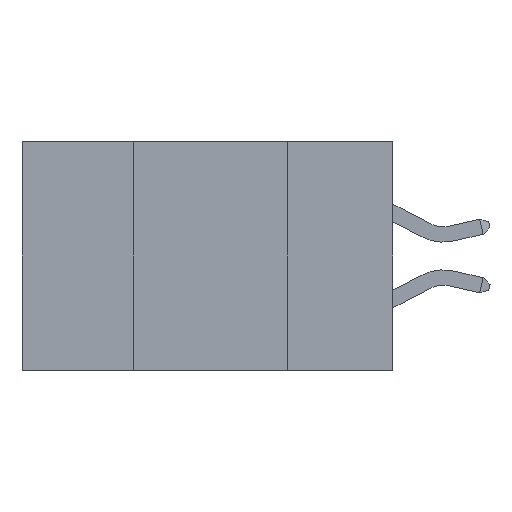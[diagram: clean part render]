
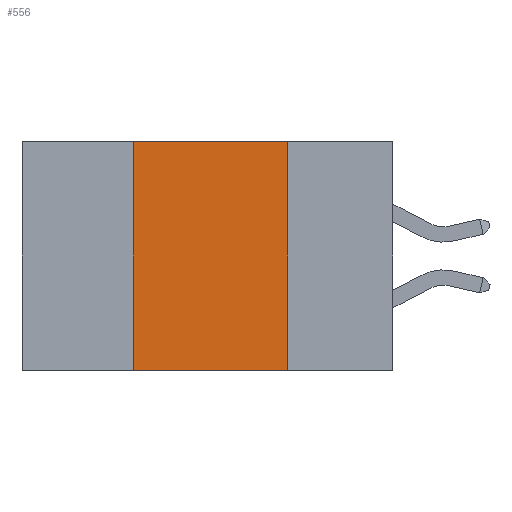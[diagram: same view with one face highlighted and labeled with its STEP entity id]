
A CAD part, left-side view. The second image highlights one B-rep face of the part: STEP entity #556.
In plain terms, the highlighted planar face has unit normal (-1, 0, 0).
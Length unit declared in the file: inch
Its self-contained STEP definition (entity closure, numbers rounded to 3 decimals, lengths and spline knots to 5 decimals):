
#556 = ADVANCED_FACE ( 'NONE', ( #12739 ), #2561, .F. ) ;
#1697 = LINE ( 'NONE', #2707, #20390 ) ;
#2165 = ORIENTED_EDGE ( 'NONE', *, *, #13111, .F. ) ;
#2561 = PLANE ( 'NONE',  #3163 ) ;
#2707 = CARTESIAN_POINT ( 'NONE',  ( 0., 0.17, 0. ) ) ;
#3163 = AXIS2_PLACEMENT_3D ( 'NONE', #14183, #4219, #16128 ) ;
#3192 = CARTESIAN_POINT ( 'NONE',  ( 0., 0.17, -0.37 ) ) ;
#4219 = DIRECTION ( 'NONE',  ( 1., 0., 0. ) ) ;
#5098 = CARTESIAN_POINT ( 'NONE',  ( 0., 0.42, 0. ) ) ;
#5653 = DIRECTION ( 'NONE',  ( 0., -1., 0. ) ) ;
#5880 = CARTESIAN_POINT ( 'NONE',  ( 0., 0.6, -0.37 ) ) ;
#6048 = DIRECTION ( 'NONE',  ( 0., 0., -1. ) ) ;
#6660 = LINE ( 'NONE', #5880, #12620 ) ;
#6897 = VECTOR ( 'NONE', #8496, 39.37008 ) ;
#8496 = DIRECTION ( 'NONE',  ( 0., 0., 1. ) ) ;
#9230 = VERTEX_POINT ( 'NONE', #3192 ) ;
#9421 = CARTESIAN_POINT ( 'NONE',  ( 0., 0.42, -0.37 ) ) ;
#11827 = EDGE_CURVE ( 'NONE', #20828, #9230, #1697, .T. ) ;
#11989 = VERTEX_POINT ( 'NONE', #9421 ) ;
#12106 = VERTEX_POINT ( 'NONE', #5098 ) ;
#12620 = VECTOR ( 'NONE', #5653, 39.37008 ) ;
#12739 = FACE_OUTER_BOUND ( 'NONE', #16812, .T. ) ;
#13111 = EDGE_CURVE ( 'NONE', #12106, #20828, #16442, .T. ) ;
#14183 = CARTESIAN_POINT ( 'NONE',  ( 0., 0.6, 0. ) ) ;
#16128 = DIRECTION ( 'NONE',  ( 0., 0., -1. ) ) ;
#16189 = DIRECTION ( 'NONE',  ( 0., -1., 0. ) ) ;
#16442 = LINE ( 'NONE', #17753, #16701 ) ;
#16701 = VECTOR ( 'NONE', #16189, 39.37008 ) ;
#16812 = EDGE_LOOP ( 'NONE', ( #17269, #2165, #16957, #21426 ) ) ;
#16957 = ORIENTED_EDGE ( 'NONE', *, *, #18823, .F. ) ;
#16996 = LINE ( 'NONE', #20209, #6897 ) ;
#17269 = ORIENTED_EDGE ( 'NONE', *, *, #11827, .F. ) ;
#17753 = CARTESIAN_POINT ( 'NONE',  ( 0., 0.6, 0. ) ) ;
#17919 = EDGE_CURVE ( 'NONE', #11989, #9230, #6660, .T. ) ;
#18823 = EDGE_CURVE ( 'NONE', #11989, #12106, #16996, .T. ) ;
#20209 = CARTESIAN_POINT ( 'NONE',  ( 0., 0.42, 0. ) ) ;
#20275 = CARTESIAN_POINT ( 'NONE',  ( 0., 0.17, 0. ) ) ;
#20390 = VECTOR ( 'NONE', #6048, 39.37008 ) ;
#20828 = VERTEX_POINT ( 'NONE', #20275 ) ;
#21426 = ORIENTED_EDGE ( 'NONE', *, *, #17919, .T. ) ;
